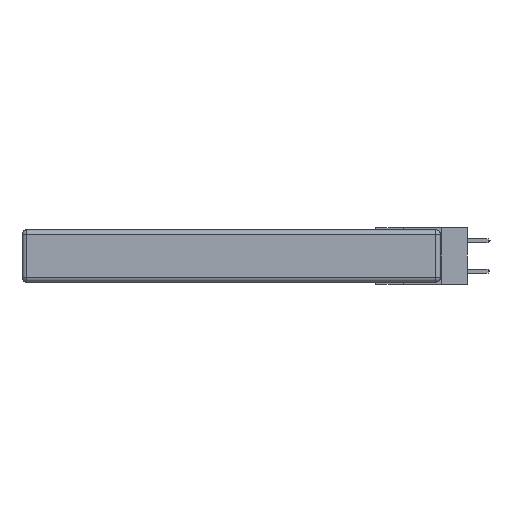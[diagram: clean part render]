
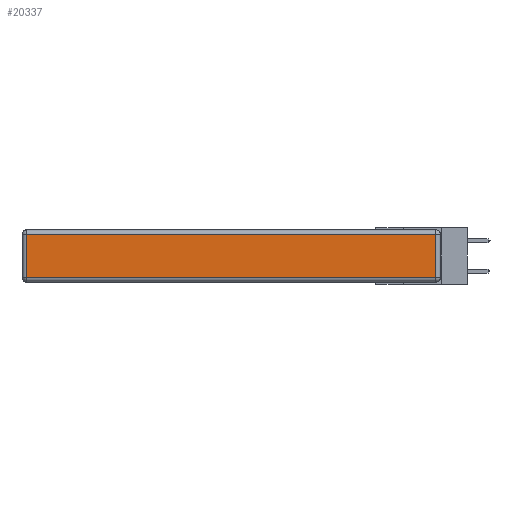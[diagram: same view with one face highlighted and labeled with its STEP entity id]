
A CAD part, left-side view. The second image highlights one B-rep face of the part: STEP entity #20337.
In plain terms, the highlighted planar face has unit normal (-1, 0, 0).
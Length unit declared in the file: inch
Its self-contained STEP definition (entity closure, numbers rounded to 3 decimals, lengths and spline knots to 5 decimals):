
#1664 = CARTESIAN_POINT ( 'NONE',  ( 0., 0.03, -0.313 ) ) ;
#1744 = VECTOR ( 'NONE', #3762, 39.37008 ) ;
#1852 = CARTESIAN_POINT ( 'NONE',  ( 0., 2.72, -0.03 ) ) ;
#3000 = EDGE_LOOP ( 'NONE', ( #15723, #8618, #10306, #10388 ) ) ;
#3191 = CARTESIAN_POINT ( 'NONE',  ( 0., 2.75, -0.03 ) ) ;
#3261 = VERTEX_POINT ( 'NONE', #1664 ) ;
#3762 = DIRECTION ( 'NONE',  ( 0., -1., 0. ) ) ;
#3786 = CARTESIAN_POINT ( 'NONE',  ( 0., 2.72, -0.313 ) ) ;
#3900 = LINE ( 'NONE', #4178, #11257 ) ;
#4055 = DIRECTION ( 'NONE',  ( -1., 0., 0. ) ) ;
#4178 = CARTESIAN_POINT ( 'NONE',  ( 0., 0.03, -0.343 ) ) ;
#4915 = EDGE_CURVE ( 'NONE', #21361, #19610, #10268, .T. ) ;
#6108 = EDGE_CURVE ( 'NONE', #19610, #3261, #8800, .T. ) ;
#8333 = LINE ( 'NONE', #3191, #23156 ) ;
#8437 = AXIS2_PLACEMENT_3D ( 'NONE', #10707, #4055, #16578 ) ;
#8618 = ORIENTED_EDGE ( 'NONE', *, *, #15038, .T. ) ;
#8800 = LINE ( 'NONE', #16500, #1744 ) ;
#10268 = LINE ( 'NONE', #13933, #13913 ) ;
#10306 = ORIENTED_EDGE ( 'NONE', *, *, #20698, .T. ) ;
#10388 = ORIENTED_EDGE ( 'NONE', *, *, #4915, .T. ) ;
#10707 = CARTESIAN_POINT ( 'NONE',  ( 0., 0., -0.343 ) ) ;
#10866 = PLANE ( 'NONE',  #8437 ) ;
#11257 = VECTOR ( 'NONE', #15129, 39.37008 ) ;
#12263 = FACE_OUTER_BOUND ( 'NONE', #3000, .T. ) ;
#13858 = DIRECTION ( 'NONE',  ( 0., 0., -1. ) ) ;
#13913 = VECTOR ( 'NONE', #13858, 39.37008 ) ;
#13933 = CARTESIAN_POINT ( 'NONE',  ( 0., 2.72, -0.343 ) ) ;
#15038 = EDGE_CURVE ( 'NONE', #3261, #23229, #3900, .T. ) ;
#15129 = DIRECTION ( 'NONE',  ( 0., 0., 1. ) ) ;
#15723 = ORIENTED_EDGE ( 'NONE', *, *, #6108, .T. ) ;
#15851 = DIRECTION ( 'NONE',  ( 0., 1., 0. ) ) ;
#16500 = CARTESIAN_POINT ( 'NONE',  ( 0., 0., -0.313 ) ) ;
#16578 = DIRECTION ( 'NONE',  ( 0., 0., 1. ) ) ;
#17308 = CARTESIAN_POINT ( 'NONE',  ( 0., 0.03, -0.03 ) ) ;
#19610 = VERTEX_POINT ( 'NONE', #3786 ) ;
#20337 = ADVANCED_FACE ( 'NONE', ( #12263 ), #10866, .T. ) ;
#20698 = EDGE_CURVE ( 'NONE', #23229, #21361, #8333, .T. ) ;
#21361 = VERTEX_POINT ( 'NONE', #1852 ) ;
#23156 = VECTOR ( 'NONE', #15851, 39.37008 ) ;
#23229 = VERTEX_POINT ( 'NONE', #17308 ) ;
